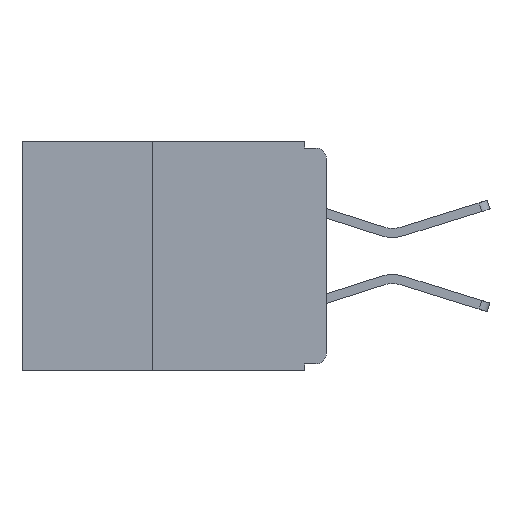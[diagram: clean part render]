
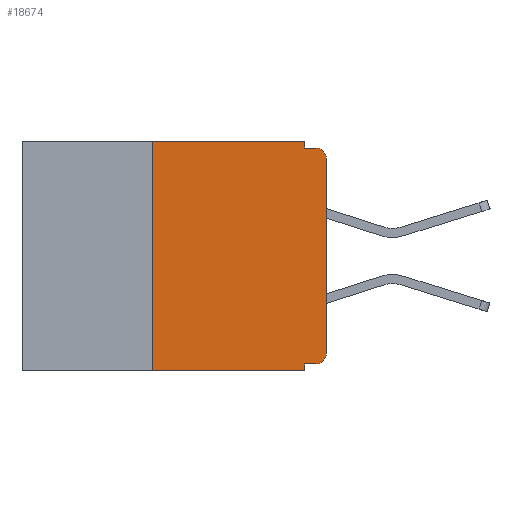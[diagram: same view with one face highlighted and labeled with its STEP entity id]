
A CAD part, left-side view. The second image highlights one B-rep face of the part: STEP entity #18674.
In plain terms, the highlighted planar face has unit normal (-1, 0, 0).
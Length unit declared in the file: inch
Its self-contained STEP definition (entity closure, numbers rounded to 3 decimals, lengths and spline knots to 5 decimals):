
#91 = CARTESIAN_POINT ( 'NONE',  ( 0., 0.25, -0.33 ) ) ;
#380 = VERTEX_POINT ( 'NONE', #16034 ) ;
#887 = CIRCLE ( 'NONE', #6480, 0.015 ) ;
#895 = CARTESIAN_POINT ( 'NONE',  ( 0., 0.015, -0.01 ) ) ;
#1096 = CIRCLE ( 'NONE', #13534, 0.015 ) ;
#1318 = VECTOR ( 'NONE', #23878, 39.37008 ) ;
#1725 = DIRECTION ( 'NONE',  ( 0., -1., 0. ) ) ;
#1891 = VECTOR ( 'NONE', #3076, 39.37008 ) ;
#1995 = CARTESIAN_POINT ( 'NONE',  ( 0., 0., -0.305 ) ) ;
#2009 = LINE ( 'NONE', #21864, #1318 ) ;
#2035 = LINE ( 'NONE', #3170, #21663 ) ;
#2381 = EDGE_CURVE ( 'NONE', #12827, #13344, #887, .T. ) ;
#2834 = DIRECTION ( 'NONE',  ( 0., 0., -1. ) ) ;
#3076 = DIRECTION ( 'NONE',  ( 0., 1., 0. ) ) ;
#3114 = CARTESIAN_POINT ( 'NONE',  ( 0., 0., -0.32 ) ) ;
#3170 = CARTESIAN_POINT ( 'NONE',  ( 0., 0.031, -0.33 ) ) ;
#3450 = ORIENTED_EDGE ( 'NONE', *, *, #6802, .F. ) ;
#3469 = VERTEX_POINT ( 'NONE', #91 ) ;
#3919 = DIRECTION ( 'NONE',  ( 0., -1., 0. ) ) ;
#4223 = VECTOR ( 'NONE', #24228, 39.37008 ) ;
#4293 = ORIENTED_EDGE ( 'NONE', *, *, #9515, .F. ) ;
#4699 = VECTOR ( 'NONE', #1725, 39.37008 ) ;
#4747 = ORIENTED_EDGE ( 'NONE', *, *, #12176, .F. ) ;
#5273 = EDGE_CURVE ( 'NONE', #18874, #12556, #1096, .T. ) ;
#5311 = DIRECTION ( 'NONE',  ( 0., 0., 1. ) ) ;
#6085 = VECTOR ( 'NONE', #3919, 39.37008 ) ;
#6480 = AXIS2_PLACEMENT_3D ( 'NONE', #15308, #15287, #15222 ) ;
#6802 = EDGE_CURVE ( 'NONE', #17483, #16931, #2035, .T. ) ;
#7107 = CARTESIAN_POINT ( 'NONE',  ( 0., 0.437, 0. ) ) ;
#7988 = EDGE_CURVE ( 'NONE', #12827, #17483, #13418, .T. ) ;
#8144 = EDGE_CURVE ( 'NONE', #3469, #16931, #15563, .T. ) ;
#8709 = VERTEX_POINT ( 'NONE', #14068 ) ;
#9128 = DIRECTION ( 'NONE',  ( 1., 0., 0. ) ) ;
#9515 = EDGE_CURVE ( 'NONE', #3469, #380, #18634, .T. ) ;
#10023 = CARTESIAN_POINT ( 'NONE',  ( 0., 0., -0.01 ) ) ;
#10155 = LINE ( 'NONE', #10023, #4699 ) ;
#10744 = ORIENTED_EDGE ( 'NONE', *, *, #5273, .T. ) ;
#11370 = VERTEX_POINT ( 'NONE', #19442 ) ;
#11441 = LINE ( 'NONE', #24047, #6085 ) ;
#12176 = EDGE_CURVE ( 'NONE', #8709, #11370, #2009, .T. ) ;
#12186 = CARTESIAN_POINT ( 'NONE',  ( 0., 0.015, -0.32 ) ) ;
#12306 = CARTESIAN_POINT ( 'NONE',  ( 0., 0.437, -0.33 ) ) ;
#12556 = VERTEX_POINT ( 'NONE', #895 ) ;
#12738 = DIRECTION ( 'NONE',  ( 0., 0., 1. ) ) ;
#12796 = LINE ( 'NONE', #17216, #22145 ) ;
#12827 = VERTEX_POINT ( 'NONE', #12186 ) ;
#13344 = VERTEX_POINT ( 'NONE', #1995 ) ;
#13376 = VECTOR ( 'NONE', #12738, 39.37008 ) ;
#13418 = LINE ( 'NONE', #3114, #1891 ) ;
#13534 = AXIS2_PLACEMENT_3D ( 'NONE', #21704, #21332, #21249 ) ;
#13820 = ORIENTED_EDGE ( 'NONE', *, *, #14177, .F. ) ;
#14068 = CARTESIAN_POINT ( 'NONE',  ( 0., 0.031, 0. ) ) ;
#14177 = EDGE_CURVE ( 'NONE', #380, #8709, #11441, .T. ) ;
#14638 = EDGE_CURVE ( 'NONE', #11370, #12556, #10155, .T. ) ;
#15061 = EDGE_LOOP ( 'NONE', ( #16777, #10744, #21887, #4747, #13820, #4293, #16880, #3450, #21022, #23185 ) ) ;
#15222 = DIRECTION ( 'NONE',  ( 0., 0., -1. ) ) ;
#15287 = DIRECTION ( 'NONE',  ( -1., 0., 0. ) ) ;
#15308 = CARTESIAN_POINT ( 'NONE',  ( 0., 0.015, -0.305 ) ) ;
#15563 = LINE ( 'NONE', #12306, #4223 ) ;
#15576 = CARTESIAN_POINT ( 'NONE',  ( 0., 0.031, -0.32 ) ) ;
#16034 = CARTESIAN_POINT ( 'NONE',  ( 0., 0.25, 0. ) ) ;
#16777 = ORIENTED_EDGE ( 'NONE', *, *, #16860, .T. ) ;
#16860 = EDGE_CURVE ( 'NONE', #13344, #18874, #12796, .T. ) ;
#16880 = ORIENTED_EDGE ( 'NONE', *, *, #8144, .T. ) ;
#16931 = VERTEX_POINT ( 'NONE', #17485 ) ;
#17216 = CARTESIAN_POINT ( 'NONE',  ( 0., 0., 0. ) ) ;
#17483 = VERTEX_POINT ( 'NONE', #15576 ) ;
#17485 = CARTESIAN_POINT ( 'NONE',  ( 0., 0.031, -0.33 ) ) ;
#18634 = LINE ( 'NONE', #22577, #13376 ) ;
#18674 = ADVANCED_FACE ( 'NONE', ( #21147 ), #19003, .F. ) ;
#18874 = VERTEX_POINT ( 'NONE', #21731 ) ;
#19003 = PLANE ( 'NONE',  #23124 ) ;
#19442 = CARTESIAN_POINT ( 'NONE',  ( 0., 0.031, -0.01 ) ) ;
#21022 = ORIENTED_EDGE ( 'NONE', *, *, #7988, .F. ) ;
#21147 = FACE_OUTER_BOUND ( 'NONE', #15061, .T. ) ;
#21249 = DIRECTION ( 'NONE',  ( 0., 0., -1. ) ) ;
#21332 = DIRECTION ( 'NONE',  ( -1., 0., 0. ) ) ;
#21663 = VECTOR ( 'NONE', #2834, 39.37008 ) ;
#21704 = CARTESIAN_POINT ( 'NONE',  ( 0., 0.015, -0.025 ) ) ;
#21731 = CARTESIAN_POINT ( 'NONE',  ( 0., 0., -0.025 ) ) ;
#21864 = CARTESIAN_POINT ( 'NONE',  ( 0., 0.031, 0. ) ) ;
#21887 = ORIENTED_EDGE ( 'NONE', *, *, #14638, .F. ) ;
#22145 = VECTOR ( 'NONE', #5311, 39.37008 ) ;
#22577 = CARTESIAN_POINT ( 'NONE',  ( 0., 0.25, -0.33 ) ) ;
#23046 = DIRECTION ( 'NONE',  ( 0., 0., -1. ) ) ;
#23124 = AXIS2_PLACEMENT_3D ( 'NONE', #7107, #9128, #23046 ) ;
#23185 = ORIENTED_EDGE ( 'NONE', *, *, #2381, .T. ) ;
#23878 = DIRECTION ( 'NONE',  ( 0., 0., -1. ) ) ;
#24047 = CARTESIAN_POINT ( 'NONE',  ( 0., 0.437, 0. ) ) ;
#24228 = DIRECTION ( 'NONE',  ( 0., -1., 0. ) ) ;
